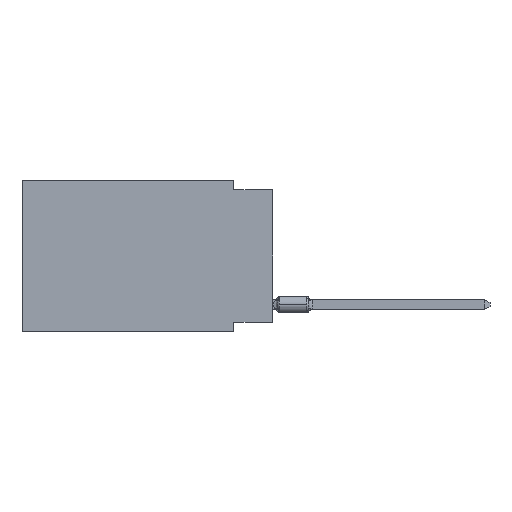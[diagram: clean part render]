
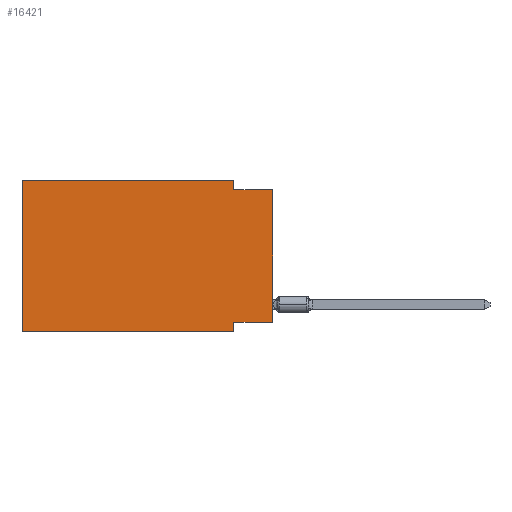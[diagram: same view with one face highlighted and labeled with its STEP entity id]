
A CAD part, left-side view. The second image highlights one B-rep face of the part: STEP entity #16421.
In plain terms, the highlighted planar face has unit normal (-1, 0, 0).
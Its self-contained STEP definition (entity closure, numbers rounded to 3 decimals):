
#252 = EDGE_CURVE ( 'NONE', #4641, #20372, #11612, .T. ) ;
#1751 = CARTESIAN_POINT ( 'NONE',  ( 0., 2.54, -9.271 ) ) ;
#2118 = CARTESIAN_POINT ( 'NONE',  ( 0., 16.383, 0. ) ) ;
#2143 = DIRECTION ( 'NONE',  ( 0., -1., 0. ) ) ;
#2426 = VERTEX_POINT ( 'NONE', #9796 ) ;
#3413 = LINE ( 'NONE', #26183, #19823 ) ;
#3531 = ORIENTED_EDGE ( 'NONE', *, *, #20853, .F. ) ;
#4354 = VECTOR ( 'NONE', #13249, 1000. ) ;
#4641 = VERTEX_POINT ( 'NONE', #1751 ) ;
#4844 = AXIS2_PLACEMENT_3D ( 'NONE', #13234, #14986, #15117 ) ;
#5275 = VECTOR ( 'NONE', #25030, 1000. ) ;
#5370 = LINE ( 'NONE', #21301, #4354 ) ;
#5918 = CARTESIAN_POINT ( 'NONE',  ( 0., 16.383, -9.906 ) ) ;
#5941 = EDGE_CURVE ( 'NONE', #2426, #6076, #8598, .T. ) ;
#6076 = VERTEX_POINT ( 'NONE', #13524 ) ;
#7571 = ORIENTED_EDGE ( 'NONE', *, *, #19239, .F. ) ;
#7810 = VECTOR ( 'NONE', #12705, 1000. ) ;
#8598 = LINE ( 'NONE', #17294, #19158 ) ;
#9380 = VERTEX_POINT ( 'NONE', #12055 ) ;
#9796 = CARTESIAN_POINT ( 'NONE',  ( 0., 2.54, 0. ) ) ;
#10509 = VERTEX_POINT ( 'NONE', #5918 ) ;
#10582 = LINE ( 'NONE', #2118, #7810 ) ;
#10970 = PLANE ( 'NONE',  #4844 ) ;
#11056 = CARTESIAN_POINT ( 'NONE',  ( 0., 16.383, 0. ) ) ;
#11612 = LINE ( 'NONE', #14010, #24331 ) ;
#12055 = CARTESIAN_POINT ( 'NONE',  ( 0., 0., -0.635 ) ) ;
#12309 = CARTESIAN_POINT ( 'NONE',  ( 0., 0., 0. ) ) ;
#12705 = DIRECTION ( 'NONE',  ( 0., -1., 0. ) ) ;
#12813 = ORIENTED_EDGE ( 'NONE', *, *, #252, .F. ) ;
#13234 = CARTESIAN_POINT ( 'NONE',  ( 0., 16.383, 0. ) ) ;
#13249 = DIRECTION ( 'NONE',  ( 0., 1., 0. ) ) ;
#13524 = CARTESIAN_POINT ( 'NONE',  ( 0., 2.54, -0.635 ) ) ;
#14010 = CARTESIAN_POINT ( 'NONE',  ( 0., 2.54, -9.906 ) ) ;
#14986 = DIRECTION ( 'NONE',  ( 1., 0., 0. ) ) ;
#15117 = DIRECTION ( 'NONE',  ( 0., 0., -1. ) ) ;
#15249 = FACE_OUTER_BOUND ( 'NONE', #18570, .T. ) ;
#15385 = VECTOR ( 'NONE', #18952, 1000. ) ;
#16015 = ORIENTED_EDGE ( 'NONE', *, *, #17556, .F. ) ;
#16344 = ORIENTED_EDGE ( 'NONE', *, *, #5941, .F. ) ;
#16421 = ADVANCED_FACE ( 'NONE', ( #15249 ), #10970, .F. ) ;
#16846 = LINE ( 'NONE', #12309, #5275 ) ;
#17294 = CARTESIAN_POINT ( 'NONE',  ( 0., 2.54, 0. ) ) ;
#17556 = EDGE_CURVE ( 'NONE', #22704, #2426, #10582, .T. ) ;
#18570 = EDGE_LOOP ( 'NONE', ( #19079, #25904, #16344, #16015, #7571, #22295, #12813, #3531 ) ) ;
#18931 = VECTOR ( 'NONE', #2143, 1000. ) ;
#18952 = DIRECTION ( 'NONE',  ( 0., -1., 0. ) ) ;
#19079 = ORIENTED_EDGE ( 'NONE', *, *, #26103, .T. ) ;
#19158 = VECTOR ( 'NONE', #20914, 1000. ) ;
#19166 = VERTEX_POINT ( 'NONE', #19364 ) ;
#19239 = EDGE_CURVE ( 'NONE', #10509, #22704, #3413, .T. ) ;
#19364 = CARTESIAN_POINT ( 'NONE',  ( 0., 0., -9.271 ) ) ;
#19823 = VECTOR ( 'NONE', #23658, 1000. ) ;
#20238 = CARTESIAN_POINT ( 'NONE',  ( 0., 0., -0.635 ) ) ;
#20372 = VERTEX_POINT ( 'NONE', #24364 ) ;
#20374 = LINE ( 'NONE', #20238, #18931 ) ;
#20577 = LINE ( 'NONE', #24989, #15385 ) ;
#20668 = EDGE_CURVE ( 'NONE', #6076, #9380, #20374, .T. ) ;
#20853 = EDGE_CURVE ( 'NONE', #19166, #4641, #5370, .T. ) ;
#20914 = DIRECTION ( 'NONE',  ( 0., 0., -1. ) ) ;
#21301 = CARTESIAN_POINT ( 'NONE',  ( 0., 0., -9.271 ) ) ;
#21800 = DIRECTION ( 'NONE',  ( 0., 0., -1. ) ) ;
#22295 = ORIENTED_EDGE ( 'NONE', *, *, #22491, .T. ) ;
#22491 = EDGE_CURVE ( 'NONE', #10509, #20372, #20577, .T. ) ;
#22704 = VERTEX_POINT ( 'NONE', #11056 ) ;
#23658 = DIRECTION ( 'NONE',  ( 0., 0., 1. ) ) ;
#24331 = VECTOR ( 'NONE', #21800, 1000. ) ;
#24364 = CARTESIAN_POINT ( 'NONE',  ( 0., 2.54, -9.906 ) ) ;
#24989 = CARTESIAN_POINT ( 'NONE',  ( 0., 16.383, -9.906 ) ) ;
#25030 = DIRECTION ( 'NONE',  ( 0., 0., 1. ) ) ;
#25904 = ORIENTED_EDGE ( 'NONE', *, *, #20668, .F. ) ;
#26103 = EDGE_CURVE ( 'NONE', #19166, #9380, #16846, .T. ) ;
#26183 = CARTESIAN_POINT ( 'NONE',  ( 0., 16.383, 0. ) ) ;
